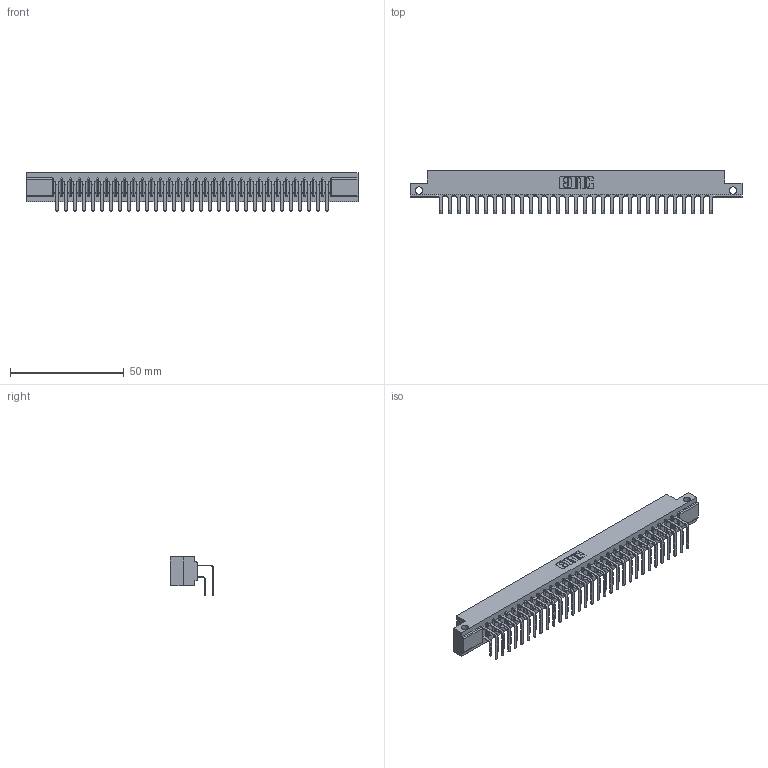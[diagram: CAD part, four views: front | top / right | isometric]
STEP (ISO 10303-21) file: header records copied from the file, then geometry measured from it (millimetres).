
FILE_DESCRIPTION (( 'STEP AP203' ), '1' );
FILE_NAME ('307-062-558-212.STEP', '2019-09-06T16:22:01', ( '' ), ( '' ), 'SwSTEP 2.0', 'SolidWorks 2016', '' );
FILE_SCHEMA (( 'CONFIG_CONTROL_DESIGN' ));
Length unit declared in the file: inch
Products named in the file (4): 307 Part_.128 Dia Side Mounting Holes; 307-290-001_558 559 - 1 (Single); 307-062-558-212; 307-290-001_558 - 2 (Single)
Assembly tree (63 placements, depth 2):
  307-062-558-212
    307 Part_.128 Dia Side Mounting Holes
    307-290-001_558 559 - 1 (Single)  x31
    307-290-001_558 - 2 (Single)  x31
Bounding box: 145.85 x 18.96 x 16.8 mm (x, y, z)
Volume: 15563.9 mm3; surface area: 20408 mm2
Topology: 63 solids, 63 shells, 3250 faces, 9127 edges, 5914 vertices
Faces by surface type: plane 2116, cylinder 1070, sphere 64
Entity records: 30373 total; most frequent: CARTESIAN_POINT 4973, ORIENTED_EDGE 4926, DIRECTION 4875, EDGE_CURVE 2463, LINE 1883, VECTOR 1883, VERTEX_POINT 1594, AXIS2_PLACEMENT_3D 1496
